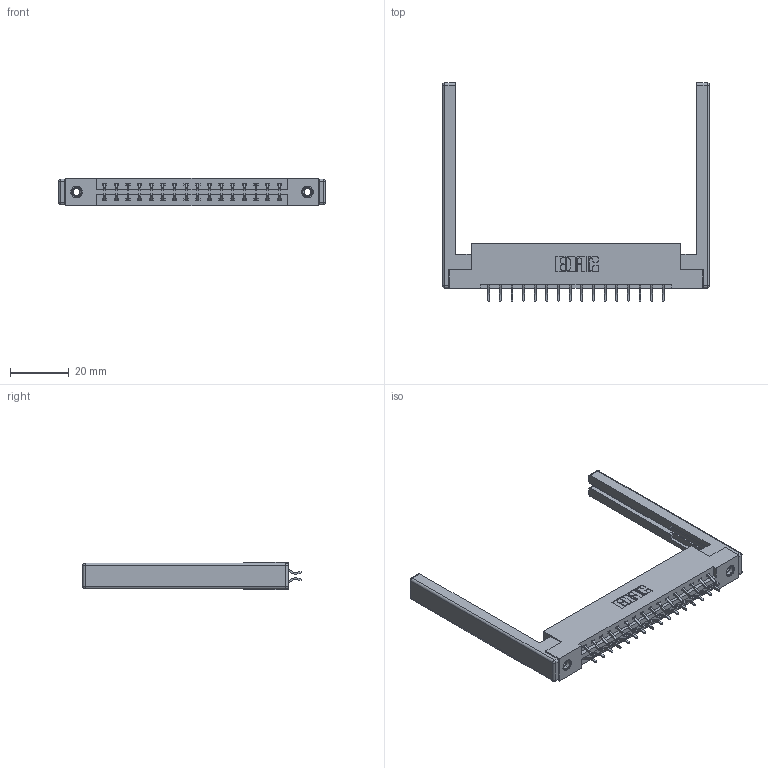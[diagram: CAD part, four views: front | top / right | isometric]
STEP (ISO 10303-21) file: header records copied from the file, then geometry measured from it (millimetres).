
FILE_DESCRIPTION (( 'STEP AP203' ), '1' );
FILE_NAME ('387-032-556-268.STEP', '2019-10-17T16:23:30', ( '' ), ( '' ), 'SwSTEP 2.0', 'SolidWorks 2016', '' );
FILE_SCHEMA (( 'CONFIG_CONTROL_DESIGN' ));
Length unit declared in the file: inch
Products named in the file (5): 307-220-068; 345-292-001_556 Tail; 337 Part_Flush Mounting Lugs - 0.156 Dia-TI; 387-032-556-268; 345-250-001_345-250-001-102
Assembly tree (37 placements, depth 2):
  387-032-556-268
    337 Part_Flush Mounting Lugs - 0.156 Dia-TI
    345-292-001_556 Tail  x32
    345-250-001_345-250-001-102  x2
    307-220-068  x2
Bounding box: 90.83 x 74.31 x 9.4 mm (x, y, z)
Volume: 13609.9 mm3; surface area: 14177 mm2
Topology: 37 solids, 37 shells, 2188 faces, 6429 edges, 4222 vertices
Faces by surface type: plane 1502, cylinder 662, cone 12, sphere 8, torus 4
Entity records: 18748 total; most frequent: CARTESIAN_POINT 3159, ORIENTED_EDGE 3072, DIRECTION 2794, EDGE_CURVE 1536, LINE 1350, VECTOR 1350, VERTEX_POINT 1014, AXIS2_PLACEMENT_3D 722
